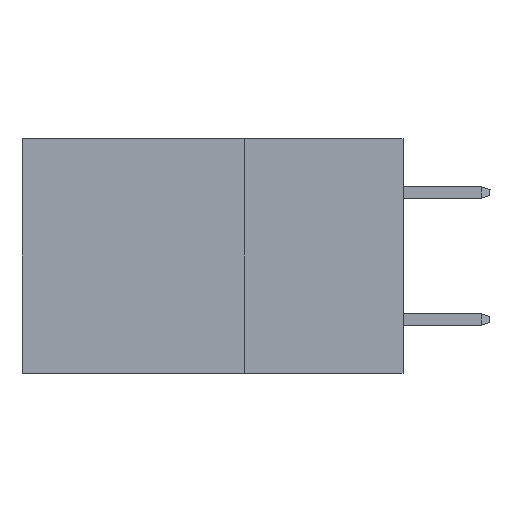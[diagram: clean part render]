
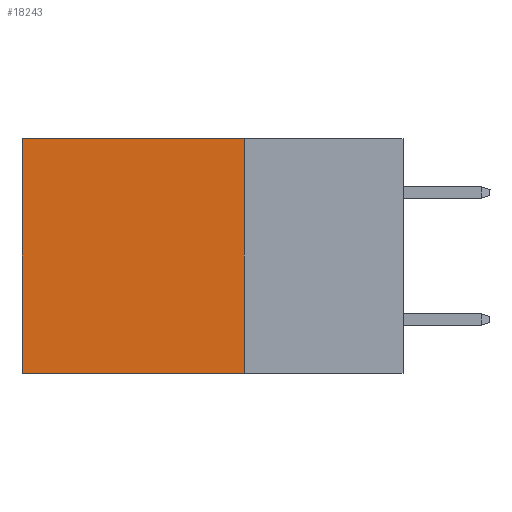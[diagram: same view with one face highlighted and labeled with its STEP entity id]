
A CAD part, left-side view. The second image highlights one B-rep face of the part: STEP entity #18243.
In plain terms, the highlighted planar face has unit normal (-1, 0, 0).
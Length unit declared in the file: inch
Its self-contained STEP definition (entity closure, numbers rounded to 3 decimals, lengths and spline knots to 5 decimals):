
#25 = CARTESIAN_POINT ( 'NONE',  ( 0.2875, 0.25, -0.37 ) ) ;
#976 = VERTEX_POINT ( 'NONE', #8598 ) ;
#2191 = LINE ( 'NONE', #8989, #19161 ) ;
#3172 = LINE ( 'NONE', #25, #17811 ) ;
#4492 = CARTESIAN_POINT ( 'NONE',  ( 0.2875, 0.6, 0. ) ) ;
#4673 = EDGE_CURVE ( 'NONE', #19324, #7642, #10120, .T. ) ;
#5061 = ORIENTED_EDGE ( 'NONE', *, *, #4673, .T. ) ;
#5336 = ORIENTED_EDGE ( 'NONE', *, *, #19397, .T. ) ;
#5714 = DIRECTION ( 'NONE',  ( 1., 0., 0. ) ) ;
#5863 = ORIENTED_EDGE ( 'NONE', *, *, #19287, .F. ) ;
#7642 = VERTEX_POINT ( 'NONE', #15532 ) ;
#8598 = CARTESIAN_POINT ( 'NONE',  ( 0.2875, 0.25, 0. ) ) ;
#8962 = ORIENTED_EDGE ( 'NONE', *, *, #16489, .F. ) ;
#8989 = CARTESIAN_POINT ( 'NONE',  ( 0.2875, 0.25, 0. ) ) ;
#10120 = LINE ( 'NONE', #4492, #10181 ) ;
#10181 = VECTOR ( 'NONE', #20422, 39.37008 ) ;
#10312 = DIRECTION ( 'NONE',  ( 0., 0., -1. ) ) ;
#10925 = VECTOR ( 'NONE', #10312, 39.37008 ) ;
#11866 = LINE ( 'NONE', #18307, #10925 ) ;
#12209 = VERTEX_POINT ( 'NONE', #20091 ) ;
#13335 = PLANE ( 'NONE',  #14312 ) ;
#13373 = DIRECTION ( 'NONE',  ( 0., 1., 0. ) ) ;
#14312 = AXIS2_PLACEMENT_3D ( 'NONE', #20070, #5714, #18500 ) ;
#14946 = CARTESIAN_POINT ( 'NONE',  ( 0.2875, 0.6, 0. ) ) ;
#15532 = CARTESIAN_POINT ( 'NONE',  ( 0.2875, 0.6, -0.37 ) ) ;
#16489 = EDGE_CURVE ( 'NONE', #976, #12209, #11866, .T. ) ;
#17811 = VECTOR ( 'NONE', #19199, 39.37008 ) ;
#18243 = ADVANCED_FACE ( 'NONE', ( #20161 ), #13335, .F. ) ;
#18307 = CARTESIAN_POINT ( 'NONE',  ( 0.2875, 0.25, 0. ) ) ;
#18500 = DIRECTION ( 'NONE',  ( 0., 0., -1. ) ) ;
#19161 = VECTOR ( 'NONE', #13373, 39.37008 ) ;
#19199 = DIRECTION ( 'NONE',  ( 0., 1., 0. ) ) ;
#19287 = EDGE_CURVE ( 'NONE', #12209, #7642, #3172, .T. ) ;
#19324 = VERTEX_POINT ( 'NONE', #14946 ) ;
#19397 = EDGE_CURVE ( 'NONE', #976, #19324, #2191, .T. ) ;
#20070 = CARTESIAN_POINT ( 'NONE',  ( 0.2875, 0.25, 0. ) ) ;
#20078 = EDGE_LOOP ( 'NONE', ( #5061, #5863, #8962, #5336 ) ) ;
#20091 = CARTESIAN_POINT ( 'NONE',  ( 0.2875, 0.25, -0.37 ) ) ;
#20161 = FACE_OUTER_BOUND ( 'NONE', #20078, .T. ) ;
#20422 = DIRECTION ( 'NONE',  ( 0., 0., -1. ) ) ;
